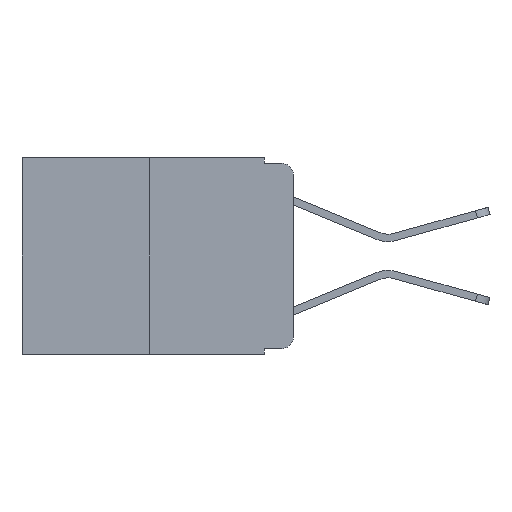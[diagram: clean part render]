
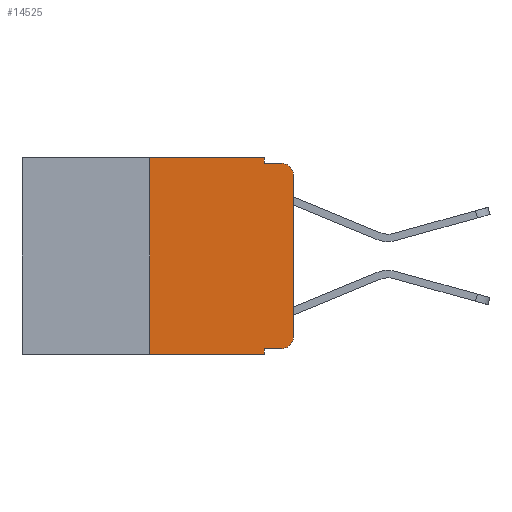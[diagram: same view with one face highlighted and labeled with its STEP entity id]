
A CAD part, left-side view. The second image highlights one B-rep face of the part: STEP entity #14525.
In plain terms, the highlighted planar face has unit normal (-1, 0, 0).
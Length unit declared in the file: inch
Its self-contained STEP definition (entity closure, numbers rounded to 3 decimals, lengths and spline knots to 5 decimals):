
#8 = EDGE_CURVE ( 'NONE', #889, #4347, #11884, .T. ) ;
#125 = EDGE_CURVE ( 'NONE', #17392, #11539, #15686, .T. ) ;
#303 = ORIENTED_EDGE ( 'NONE', *, *, #15453, .T. ) ;
#733 = VECTOR ( 'NONE', #5133, 39.37008 ) ;
#889 = VERTEX_POINT ( 'NONE', #13960 ) ;
#1241 = LINE ( 'NONE', #2915, #13407 ) ;
#1709 = DIRECTION ( 'NONE',  ( 0., -1., 0. ) ) ;
#1753 = AXIS2_PLACEMENT_3D ( 'NONE', #10724, #17553, #14287 ) ;
#2015 = EDGE_CURVE ( 'NONE', #11077, #8264, #12460, .T. ) ;
#2019 = VECTOR ( 'NONE', #3934, 39.37008 ) ;
#2116 = EDGE_CURVE ( 'NONE', #8115, #11077, #7971, .T. ) ;
#2573 = ORIENTED_EDGE ( 'NONE', *, *, #11981, .T. ) ;
#2915 = CARTESIAN_POINT ( 'NONE',  ( 0., 0.25, 0. ) ) ;
#3592 = CARTESIAN_POINT ( 'NONE',  ( 0., 0.051, 0. ) ) ;
#3645 = CARTESIAN_POINT ( 'NONE',  ( 0., 0.25, -0.343 ) ) ;
#3722 = DIRECTION ( 'NONE',  ( 0., -1., 0. ) ) ;
#3811 = CARTESIAN_POINT ( 'NONE',  ( 0., 0., 0. ) ) ;
#3855 = DIRECTION ( 'NONE',  ( 0., 0., -1. ) ) ;
#3934 = DIRECTION ( 'NONE',  ( 0., 0., -1. ) ) ;
#4094 = ORIENTED_EDGE ( 'NONE', *, *, #2116, .F. ) ;
#4347 = VERTEX_POINT ( 'NONE', #19370 ) ;
#4436 = ORIENTED_EDGE ( 'NONE', *, *, #21981, .T. ) ;
#4480 = ORIENTED_EDGE ( 'NONE', *, *, #8, .T. ) ;
#5131 = CARTESIAN_POINT ( 'NONE',  ( 0., 0.051, -0.343 ) ) ;
#5133 = DIRECTION ( 'NONE',  ( 0., 0., -1. ) ) ;
#5670 = CIRCLE ( 'NONE', #1753, 0.02 ) ;
#6855 = LINE ( 'NONE', #11994, #18314 ) ;
#7090 = LINE ( 'NONE', #13914, #21052 ) ;
#7206 = VECTOR ( 'NONE', #1709, 39.37008 ) ;
#7235 = CARTESIAN_POINT ( 'NONE',  ( 0., 0.473, 0. ) ) ;
#7623 = EDGE_CURVE ( 'NONE', #16890, #8115, #1241, .T. ) ;
#7650 = CARTESIAN_POINT ( 'NONE',  ( 0., 0., -0.313 ) ) ;
#7971 = LINE ( 'NONE', #14793, #17401 ) ;
#8115 = VERTEX_POINT ( 'NONE', #10051 ) ;
#8246 = CIRCLE ( 'NONE', #20794, 0.02 ) ;
#8264 = VERTEX_POINT ( 'NONE', #15748 ) ;
#9089 = DIRECTION ( 'NONE',  ( 0., 0., 1. ) ) ;
#9726 = ORIENTED_EDGE ( 'NONE', *, *, #125, .T. ) ;
#10051 = CARTESIAN_POINT ( 'NONE',  ( 0., 0.25, 0. ) ) ;
#10319 = ORIENTED_EDGE ( 'NONE', *, *, #2015, .F. ) ;
#10712 = PLANE ( 'NONE',  #20383 ) ;
#10724 = CARTESIAN_POINT ( 'NONE',  ( 0., 0.02, -0.03 ) ) ;
#10839 = ORIENTED_EDGE ( 'NONE', *, *, #7623, .F. ) ;
#10985 = CARTESIAN_POINT ( 'NONE',  ( 0., 0.051, 0. ) ) ;
#11061 = CARTESIAN_POINT ( 'NONE',  ( 0., 0.02, -0.01 ) ) ;
#11077 = VERTEX_POINT ( 'NONE', #10985 ) ;
#11098 = DIRECTION ( 'NONE',  ( 0., 0., 1. ) ) ;
#11177 = DIRECTION ( 'NONE',  ( -1., 0., 0. ) ) ;
#11539 = VERTEX_POINT ( 'NONE', #16312 ) ;
#11884 = LINE ( 'NONE', #18746, #7206 ) ;
#11981 = EDGE_CURVE ( 'NONE', #16890, #15153, #7090, .T. ) ;
#11994 = CARTESIAN_POINT ( 'NONE',  ( 0., 0.051, -0.01 ) ) ;
#12460 = LINE ( 'NONE', #19303, #2019 ) ;
#13407 = VECTOR ( 'NONE', #11098, 39.37008 ) ;
#13914 = CARTESIAN_POINT ( 'NONE',  ( 0., 0.473, -0.343 ) ) ;
#13960 = CARTESIAN_POINT ( 'NONE',  ( 0., 0.051, -0.333 ) ) ;
#14287 = DIRECTION ( 'NONE',  ( 0., 0., -1. ) ) ;
#14525 = ADVANCED_FACE ( 'NONE', ( #15511 ), #10712, .F. ) ;
#14793 = CARTESIAN_POINT ( 'NONE',  ( 0., 0.473, 0. ) ) ;
#15153 = VERTEX_POINT ( 'NONE', #5131 ) ;
#15453 = EDGE_CURVE ( 'NONE', #4347, #17392, #8246, .T. ) ;
#15511 = FACE_OUTER_BOUND ( 'NONE', #19166, .T. ) ;
#15531 = ORIENTED_EDGE ( 'NONE', *, *, #20227, .F. ) ;
#15686 = LINE ( 'NONE', #3811, #18654 ) ;
#15748 = CARTESIAN_POINT ( 'NONE',  ( 0., 0.051, -0.01 ) ) ;
#16312 = CARTESIAN_POINT ( 'NONE',  ( 0., 0., -0.03 ) ) ;
#16890 = VERTEX_POINT ( 'NONE', #3645 ) ;
#17392 = VERTEX_POINT ( 'NONE', #7650 ) ;
#17401 = VECTOR ( 'NONE', #19752, 39.37008 ) ;
#17553 = DIRECTION ( 'NONE',  ( -1., 0., 0. ) ) ;
#18124 = CARTESIAN_POINT ( 'NONE',  ( 0., 0.02, -0.313 ) ) ;
#18314 = VECTOR ( 'NONE', #18958, 39.37008 ) ;
#18525 = ORIENTED_EDGE ( 'NONE', *, *, #21449, .F. ) ;
#18654 = VECTOR ( 'NONE', #9089, 39.37008 ) ;
#18746 = CARTESIAN_POINT ( 'NONE',  ( 0., 0.051, -0.333 ) ) ;
#18958 = DIRECTION ( 'NONE',  ( 0., -1., 0. ) ) ;
#19027 = VERTEX_POINT ( 'NONE', #11061 ) ;
#19166 = EDGE_LOOP ( 'NONE', ( #9726, #4436, #18525, #10319, #4094, #10839, #2573, #15531, #4480, #303 ) ) ;
#19303 = CARTESIAN_POINT ( 'NONE',  ( 0., 0.051, 0. ) ) ;
#19370 = CARTESIAN_POINT ( 'NONE',  ( 0., 0.02, -0.333 ) ) ;
#19752 = DIRECTION ( 'NONE',  ( 0., -1., 0. ) ) ;
#20227 = EDGE_CURVE ( 'NONE', #889, #15153, #21972, .T. ) ;
#20383 = AXIS2_PLACEMENT_3D ( 'NONE', #7235, #20694, #3855 ) ;
#20694 = DIRECTION ( 'NONE',  ( 1., 0., 0. ) ) ;
#20794 = AXIS2_PLACEMENT_3D ( 'NONE', #18124, #11177, #21823 ) ;
#21052 = VECTOR ( 'NONE', #3722, 39.37008 ) ;
#21449 = EDGE_CURVE ( 'NONE', #8264, #19027, #6855, .T. ) ;
#21823 = DIRECTION ( 'NONE',  ( 0., 0., -1. ) ) ;
#21972 = LINE ( 'NONE', #3592, #733 ) ;
#21981 = EDGE_CURVE ( 'NONE', #11539, #19027, #5670, .T. ) ;
